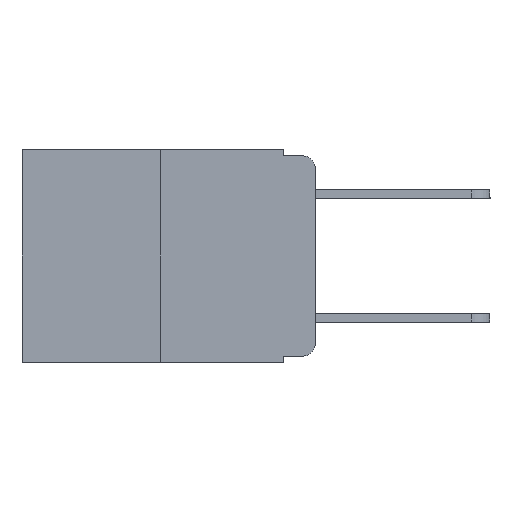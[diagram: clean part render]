
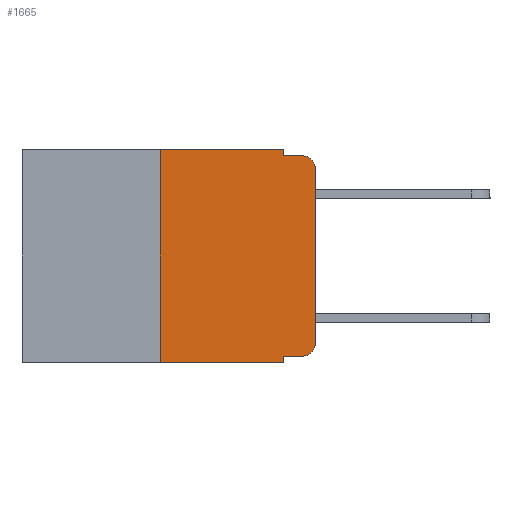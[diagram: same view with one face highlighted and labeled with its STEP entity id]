
A CAD part, left-side view. The second image highlights one B-rep face of the part: STEP entity #1665.
In plain terms, the highlighted planar face has unit normal (-1, 0, 0).
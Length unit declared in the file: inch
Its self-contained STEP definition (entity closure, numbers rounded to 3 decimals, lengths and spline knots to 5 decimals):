
#234 = ORIENTED_EDGE ( 'NONE', *, *, #2595, .T. ) ;
#319 = LINE ( 'NONE', #950, #8194 ) ;
#450 = VERTEX_POINT ( 'NONE', #7499 ) ;
#494 = ORIENTED_EDGE ( 'NONE', *, *, #7504, .F. ) ;
#557 = ORIENTED_EDGE ( 'NONE', *, *, #6386, .T. ) ;
#593 = AXIS2_PLACEMENT_3D ( 'NONE', #8376, #2326, #1893 ) ;
#695 = ORIENTED_EDGE ( 'NONE', *, *, #6836, .F. ) ;
#787 = VECTOR ( 'NONE', #5768, 39.37008 ) ;
#950 = CARTESIAN_POINT ( 'NONE',  ( 0., 0.051, -0.01 ) ) ;
#1254 = CARTESIAN_POINT ( 'NONE',  ( 0., 0.051, -0.343 ) ) ;
#1564 = LINE ( 'NONE', #2937, #12338 ) ;
#1603 = DIRECTION ( 'NONE',  ( -1., 0., 0. ) ) ;
#1665 = ADVANCED_FACE ( 'NONE', ( #13377 ), #6891, .F. ) ;
#1680 = CARTESIAN_POINT ( 'NONE',  ( 0., 0.051, -0.333 ) ) ;
#1791 = CARTESIAN_POINT ( 'NONE',  ( 0., 0.02, -0.313 ) ) ;
#1893 = DIRECTION ( 'NONE',  ( 0., 0., -1. ) ) ;
#2047 = CARTESIAN_POINT ( 'NONE',  ( 0., 0., -0.03 ) ) ;
#2326 = DIRECTION ( 'NONE',  ( 1., 0., 0. ) ) ;
#2595 = EDGE_CURVE ( 'NONE', #2643, #4812, #6679, .T. ) ;
#2643 = VERTEX_POINT ( 'NONE', #9874 ) ;
#2937 = CARTESIAN_POINT ( 'NONE',  ( 0., 0.25, 0. ) ) ;
#3008 = DIRECTION ( 'NONE',  ( 0., 0., -1. ) ) ;
#3127 = VERTEX_POINT ( 'NONE', #7406 ) ;
#3208 = LINE ( 'NONE', #1680, #13590 ) ;
#3256 = ORIENTED_EDGE ( 'NONE', *, *, #9081, .F. ) ;
#3484 = EDGE_CURVE ( 'NONE', #450, #9278, #10083, .T. ) ;
#3528 = ORIENTED_EDGE ( 'NONE', *, *, #3484, .T. ) ;
#3548 = ORIENTED_EDGE ( 'NONE', *, *, #9488, .T. ) ;
#4078 = DIRECTION ( 'NONE',  ( 0., -1., 0. ) ) ;
#4112 = DIRECTION ( 'NONE',  ( 0., 0., 1. ) ) ;
#4132 = VERTEX_POINT ( 'NONE', #10584 ) ;
#4244 = ORIENTED_EDGE ( 'NONE', *, *, #9828, .F. ) ;
#4274 = VECTOR ( 'NONE', #11656, 39.37008 ) ;
#4341 = LINE ( 'NONE', #11687, #787 ) ;
#4474 = VERTEX_POINT ( 'NONE', #9367 ) ;
#4716 = CIRCLE ( 'NONE', #5461, 0.02 ) ;
#4812 = VERTEX_POINT ( 'NONE', #1254 ) ;
#5180 = VERTEX_POINT ( 'NONE', #2047 ) ;
#5390 = ORIENTED_EDGE ( 'NONE', *, *, #10763, .T. ) ;
#5461 = AXIS2_PLACEMENT_3D ( 'NONE', #8205, #1603, #9171 ) ;
#5593 = VERTEX_POINT ( 'NONE', #7120 ) ;
#5768 = DIRECTION ( 'NONE',  ( 0., 0., 1. ) ) ;
#6036 = VECTOR ( 'NONE', #7413, 39.37008 ) ;
#6386 = EDGE_CURVE ( 'NONE', #5593, #450, #3208, .T. ) ;
#6679 = LINE ( 'NONE', #8741, #12172 ) ;
#6836 = EDGE_CURVE ( 'NONE', #4132, #13269, #7089, .T. ) ;
#6891 = PLANE ( 'NONE',  #593 ) ;
#7089 = LINE ( 'NONE', #11611, #4274 ) ;
#7120 = CARTESIAN_POINT ( 'NONE',  ( 0., 0.051, -0.333 ) ) ;
#7406 = CARTESIAN_POINT ( 'NONE',  ( 0., 0.02, -0.01 ) ) ;
#7413 = DIRECTION ( 'NONE',  ( 0., -1., 0. ) ) ;
#7458 = CARTESIAN_POINT ( 'NONE',  ( 0., 0.473, 0. ) ) ;
#7499 = CARTESIAN_POINT ( 'NONE',  ( 0., 0.02, -0.333 ) ) ;
#7504 = EDGE_CURVE ( 'NONE', #13269, #3127, #319, .T. ) ;
#7514 = CARTESIAN_POINT ( 'NONE',  ( 0., 0.051, -0.01 ) ) ;
#7633 = CARTESIAN_POINT ( 'NONE',  ( 0., 0.051, 0. ) ) ;
#7905 = CARTESIAN_POINT ( 'NONE',  ( 0., 0., -0.313 ) ) ;
#8194 = VECTOR ( 'NONE', #13415, 39.37008 ) ;
#8205 = CARTESIAN_POINT ( 'NONE',  ( 0., 0.02, -0.03 ) ) ;
#8263 = DIRECTION ( 'NONE',  ( 0., -1., 0. ) ) ;
#8376 = CARTESIAN_POINT ( 'NONE',  ( 0., 0.473, 0. ) ) ;
#8741 = CARTESIAN_POINT ( 'NONE',  ( 0., 0.473, -0.343 ) ) ;
#8758 = LINE ( 'NONE', #7458, #6036 ) ;
#9081 = EDGE_CURVE ( 'NONE', #5593, #4812, #12641, .T. ) ;
#9171 = DIRECTION ( 'NONE',  ( 0., 0., -1. ) ) ;
#9278 = VERTEX_POINT ( 'NONE', #7905 ) ;
#9313 = DIRECTION ( 'NONE',  ( -1., 0., 0. ) ) ;
#9367 = CARTESIAN_POINT ( 'NONE',  ( 0., 0.25, 0. ) ) ;
#9448 = EDGE_LOOP ( 'NONE', ( #5390, #3548, #494, #695, #4244, #9913, #234, #3256, #557, #3528 ) ) ;
#9488 = EDGE_CURVE ( 'NONE', #5180, #3127, #4716, .T. ) ;
#9819 = VECTOR ( 'NONE', #12445, 39.37008 ) ;
#9828 = EDGE_CURVE ( 'NONE', #4474, #4132, #8758, .T. ) ;
#9874 = CARTESIAN_POINT ( 'NONE',  ( 0., 0.25, -0.343 ) ) ;
#9913 = ORIENTED_EDGE ( 'NONE', *, *, #10371, .F. ) ;
#10083 = CIRCLE ( 'NONE', #12120, 0.02 ) ;
#10371 = EDGE_CURVE ( 'NONE', #2643, #4474, #1564, .T. ) ;
#10584 = CARTESIAN_POINT ( 'NONE',  ( 0., 0.051, 0. ) ) ;
#10763 = EDGE_CURVE ( 'NONE', #9278, #5180, #4341, .T. ) ;
#11611 = CARTESIAN_POINT ( 'NONE',  ( 0., 0.051, 0. ) ) ;
#11656 = DIRECTION ( 'NONE',  ( 0., 0., -1. ) ) ;
#11687 = CARTESIAN_POINT ( 'NONE',  ( 0., 0., 0. ) ) ;
#12120 = AXIS2_PLACEMENT_3D ( 'NONE', #1791, #9313, #3008 ) ;
#12172 = VECTOR ( 'NONE', #8263, 39.37008 ) ;
#12338 = VECTOR ( 'NONE', #4112, 39.37008 ) ;
#12445 = DIRECTION ( 'NONE',  ( 0., 0., -1. ) ) ;
#12641 = LINE ( 'NONE', #7633, #9819 ) ;
#13269 = VERTEX_POINT ( 'NONE', #7514 ) ;
#13377 = FACE_OUTER_BOUND ( 'NONE', #9448, .T. ) ;
#13415 = DIRECTION ( 'NONE',  ( 0., -1., 0. ) ) ;
#13590 = VECTOR ( 'NONE', #4078, 39.37008 ) ;
